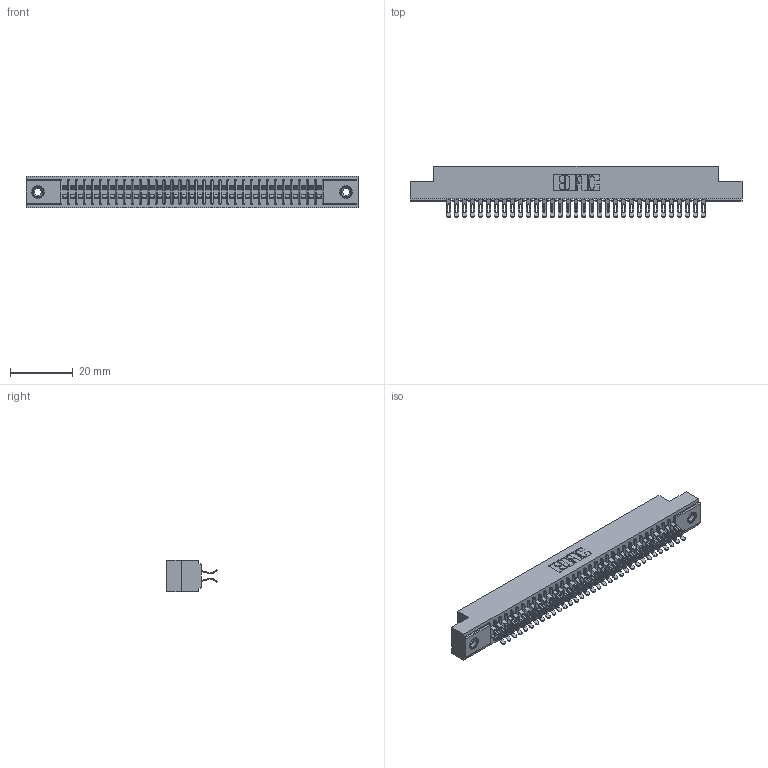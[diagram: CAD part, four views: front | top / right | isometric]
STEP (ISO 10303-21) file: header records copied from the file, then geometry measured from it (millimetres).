
FILE_DESCRIPTION (( 'STEP AP203' ), '1' );
FILE_NAME ('341-066-555-208.STEP', '2018-08-07T18:48:07', ( '' ), ( '' ), 'SwSTEP 2.0', 'SolidWorks 2016', '' );
FILE_SCHEMA (( 'CONFIG_CONTROL_DESIGN' ));
Length unit declared in the file: inch
Products named in the file (4): 341 Part_.156 (3.96) Dia Mounting Holes; 341-292-001_341-292-155; 345-250-001_345-250-003-102; 341-066-555-208
Assembly tree (69 placements, depth 2):
  341-066-555-208
    341 Part_.156 (3.96) Dia Mounting Holes
    341-292-001_341-292-155  x66
    345-250-001_345-250-003-102  x2
Bounding box: 106.05 x 16.31 x 10.16 mm (x, y, z)
Volume: 7900.3 mm3; surface area: 14297.3 mm2
Topology: 69 solids, 69 shells, 5324 faces, 15863 edges, 10322 vertices
Faces by surface type: plane 2872, cylinder 2304, sphere 68, torus 68, cone 12
Entity records: 42791 total; most frequent: CARTESIAN_POINT 7112, ORIENTED_EDGE 7050, DIRECTION 6909, EDGE_CURVE 3525, LINE 2819, VECTOR 2819, VERTEX_POINT 2232, AXIS2_PLACEMENT_3D 2045
